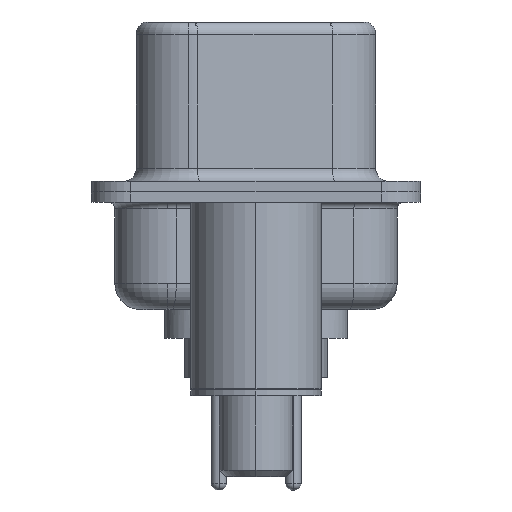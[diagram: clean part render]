
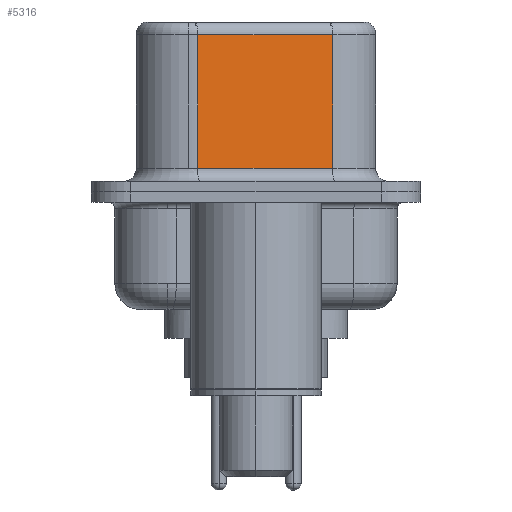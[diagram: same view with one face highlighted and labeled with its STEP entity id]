
A CAD part, left-side view. The second image highlights one B-rep face of the part: STEP entity #5316.
In plain terms, the highlighted planar face has unit normal (-0.985, -0.174, 0).
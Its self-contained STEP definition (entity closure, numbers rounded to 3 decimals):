
#2426 = EDGE_CURVE ( 'NONE', #7482, #18393, #6716, .T. ) ;
#3362 = ORIENTED_EDGE ( 'NONE', *, *, #16029, .T. ) ;
#3908 = CARTESIAN_POINT ( 'NONE',  ( 4.58, -2.927, 6.52 ) ) ;
#3949 = CARTESIAN_POINT ( 'NONE',  ( 4.58, -2.927, 6.02 ) ) ;
#4236 = VECTOR ( 'NONE', #8723, 1000. ) ;
#4473 = VECTOR ( 'NONE', #22450, 1000. ) ;
#5303 = AXIS2_PLACEMENT_3D ( 'NONE', #11619, #15828, #9596 ) ;
#5316 = ADVANCED_FACE ( 'NONE', ( #22404 ), #5850, .F. ) ;
#5460 = EDGE_LOOP ( 'NONE', ( #23659, #18324, #3362, #8764 ) ) ;
#5850 = PLANE ( 'NONE',  #5303 ) ;
#6589 = CARTESIAN_POINT ( 'NONE',  ( 3.67, 2.233, 6.52 ) ) ;
#6716 = LINE ( 'NONE', #15883, #15886 ) ;
#7482 = VERTEX_POINT ( 'NONE', #3949 ) ;
#8086 = CARTESIAN_POINT ( 'NONE',  ( 3.67, 2.233, 0.9 ) ) ;
#8273 = EDGE_CURVE ( 'NONE', #7482, #13646, #14234, .T. ) ;
#8723 = DIRECTION ( 'NONE',  ( 0.174, -0.985, 0. ) ) ;
#8764 = ORIENTED_EDGE ( 'NONE', *, *, #17436, .T. ) ;
#9596 = DIRECTION ( 'NONE',  ( -0.174, 0.985, 0. ) ) ;
#11619 = CARTESIAN_POINT ( 'NONE',  ( 4.58, -2.927, 6.52 ) ) ;
#12156 = CARTESIAN_POINT ( 'NONE',  ( 4.58, -2.927, 0.9 ) ) ;
#13646 = VERTEX_POINT ( 'NONE', #17526 ) ;
#14234 = LINE ( 'NONE', #3908, #4473 ) ;
#15544 = CARTESIAN_POINT ( 'NONE',  ( 3.67, 2.233, 6.02 ) ) ;
#15737 = DIRECTION ( 'NONE',  ( 0., 0., -1. ) ) ;
#15828 = DIRECTION ( 'NONE',  ( 0.985, 0.174, 0. ) ) ;
#15883 = CARTESIAN_POINT ( 'NONE',  ( 4.58, -2.927, 6.02 ) ) ;
#15886 = VECTOR ( 'NONE', #16907, 1000. ) ;
#16029 = EDGE_CURVE ( 'NONE', #18393, #20929, #19174, .T. ) ;
#16907 = DIRECTION ( 'NONE',  ( -0.174, 0.985, 0. ) ) ;
#17436 = EDGE_CURVE ( 'NONE', #20929, #13646, #19512, .T. ) ;
#17526 = CARTESIAN_POINT ( 'NONE',  ( 4.58, -2.927, 0.9 ) ) ;
#18324 = ORIENTED_EDGE ( 'NONE', *, *, #2426, .T. ) ;
#18393 = VERTEX_POINT ( 'NONE', #15544 ) ;
#19174 = LINE ( 'NONE', #6589, #23435 ) ;
#19512 = LINE ( 'NONE', #12156, #4236 ) ;
#20929 = VERTEX_POINT ( 'NONE', #8086 ) ;
#22404 = FACE_OUTER_BOUND ( 'NONE', #5460, .T. ) ;
#22450 = DIRECTION ( 'NONE',  ( 0., 0., -1. ) ) ;
#23435 = VECTOR ( 'NONE', #15737, 1000. ) ;
#23659 = ORIENTED_EDGE ( 'NONE', *, *, #8273, .F. ) ;
